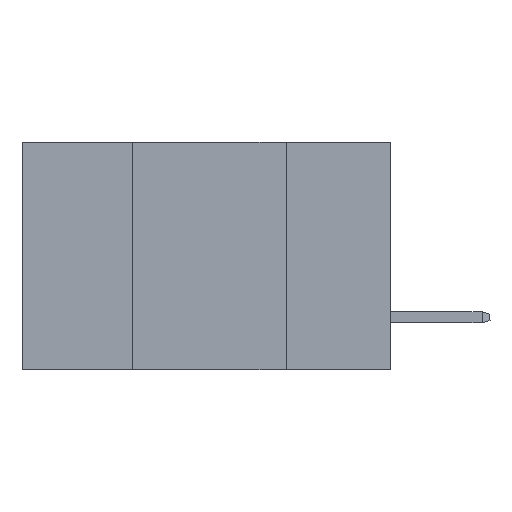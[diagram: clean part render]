
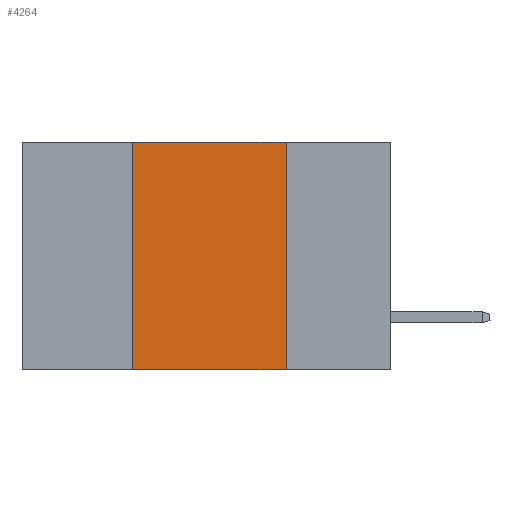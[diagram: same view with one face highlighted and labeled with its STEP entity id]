
A CAD part, left-side view. The second image highlights one B-rep face of the part: STEP entity #4264.
In plain terms, the highlighted planar face has unit normal (-1, 0, 0).
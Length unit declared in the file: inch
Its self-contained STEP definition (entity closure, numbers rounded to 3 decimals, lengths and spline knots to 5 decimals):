
#268 = CARTESIAN_POINT ( 'NONE',  ( 0., 0.17, 0. ) ) ;
#458 = EDGE_CURVE ( 'NONE', #4095, #5292, #6848, .T. ) ;
#1020 = VECTOR ( 'NONE', #10235, 39.37008 ) ;
#1032 = CARTESIAN_POINT ( 'NONE',  ( 0., 0.6, -0.37 ) ) ;
#1296 = LINE ( 'NONE', #3832, #1020 ) ;
#1497 = VECTOR ( 'NONE', #3256, 39.37008 ) ;
#2134 = CARTESIAN_POINT ( 'NONE',  ( 0., 0.42, -0.37 ) ) ;
#2621 = DIRECTION ( 'NONE',  ( 0., 0., -1. ) ) ;
#2824 = DIRECTION ( 'NONE',  ( 0., -1., 0. ) ) ;
#3256 = DIRECTION ( 'NONE',  ( 0., -1., 0. ) ) ;
#3469 = CARTESIAN_POINT ( 'NONE',  ( 0., 0.6, 0. ) ) ;
#3832 = CARTESIAN_POINT ( 'NONE',  ( 0., 0.42, 0. ) ) ;
#4095 = VERTEX_POINT ( 'NONE', #6959 ) ;
#4264 = ADVANCED_FACE ( 'NONE', ( #7980 ), #8194, .F. ) ;
#4721 = VECTOR ( 'NONE', #2824, 39.37008 ) ;
#5292 = VERTEX_POINT ( 'NONE', #6995 ) ;
#5416 = EDGE_CURVE ( 'NONE', #8295, #4095, #10501, .T. ) ;
#5463 = VERTEX_POINT ( 'NONE', #2134 ) ;
#6705 = DIRECTION ( 'NONE',  ( 0., 0., -1. ) ) ;
#6848 = LINE ( 'NONE', #268, #10573 ) ;
#6959 = CARTESIAN_POINT ( 'NONE',  ( 0., 0.17, 0. ) ) ;
#6995 = CARTESIAN_POINT ( 'NONE',  ( 0., 0.17, -0.37 ) ) ;
#7980 = FACE_OUTER_BOUND ( 'NONE', #8643, .T. ) ;
#8073 = CARTESIAN_POINT ( 'NONE',  ( 0., 0.42, 0. ) ) ;
#8094 = AXIS2_PLACEMENT_3D ( 'NONE', #9261, #8150, #6705 ) ;
#8150 = DIRECTION ( 'NONE',  ( 1., 0., 0. ) ) ;
#8165 = EDGE_CURVE ( 'NONE', #5463, #5292, #10478, .T. ) ;
#8194 = PLANE ( 'NONE',  #8094 ) ;
#8295 = VERTEX_POINT ( 'NONE', #8073 ) ;
#8643 = EDGE_LOOP ( 'NONE', ( #8792, #8992, #9038, #9100 ) ) ;
#8792 = ORIENTED_EDGE ( 'NONE', *, *, #458, .F. ) ;
#8992 = ORIENTED_EDGE ( 'NONE', *, *, #5416, .F. ) ;
#9038 = ORIENTED_EDGE ( 'NONE', *, *, #9837, .F. ) ;
#9100 = ORIENTED_EDGE ( 'NONE', *, *, #8165, .T. ) ;
#9261 = CARTESIAN_POINT ( 'NONE',  ( 0., 0.6, 0. ) ) ;
#9837 = EDGE_CURVE ( 'NONE', #5463, #8295, #1296, .T. ) ;
#10235 = DIRECTION ( 'NONE',  ( 0., 0., 1. ) ) ;
#10478 = LINE ( 'NONE', #1032, #4721 ) ;
#10501 = LINE ( 'NONE', #3469, #1497 ) ;
#10573 = VECTOR ( 'NONE', #2621, 39.37008 ) ;
